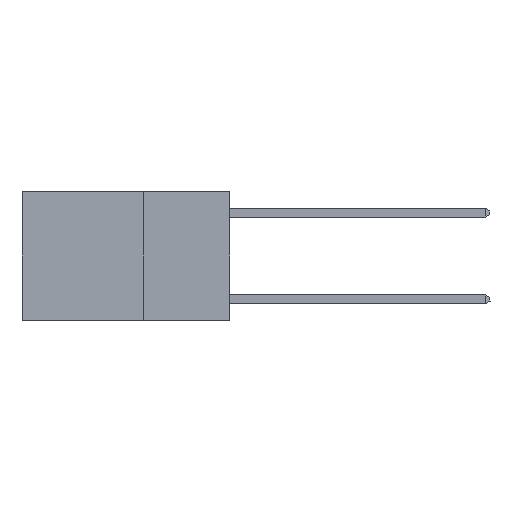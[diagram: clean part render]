
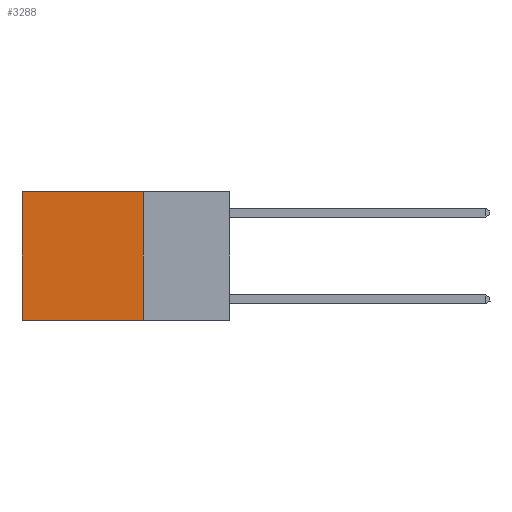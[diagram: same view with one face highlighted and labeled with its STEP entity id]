
A CAD part, left-side view. The second image highlights one B-rep face of the part: STEP entity #3288.
In plain terms, the highlighted planar face has unit normal (-1, 0, 0).
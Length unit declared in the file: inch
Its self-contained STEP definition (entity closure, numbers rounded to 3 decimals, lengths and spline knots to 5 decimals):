
#280 = CARTESIAN_POINT ( 'NONE',  ( 0.2625, 0.25, -0.37 ) ) ;
#695 = EDGE_LOOP ( 'NONE', ( #10145, #2868, #9260, #2559 ) ) ;
#1460 = LINE ( 'NONE', #3669, #13190 ) ;
#1894 = CARTESIAN_POINT ( 'NONE',  ( 0.2625, 0.6, -0.37 ) ) ;
#2559 = ORIENTED_EDGE ( 'NONE', *, *, #13387, .T. ) ;
#2843 = CARTESIAN_POINT ( 'NONE',  ( 0.2625, 0.6, 0. ) ) ;
#2868 = ORIENTED_EDGE ( 'NONE', *, *, #10816, .F. ) ;
#2948 = CARTESIAN_POINT ( 'NONE',  ( 0.2625, 0.25, -0.37 ) ) ;
#3288 = ADVANCED_FACE ( 'NONE', ( #13432 ), #14469, .F. ) ;
#3315 = CARTESIAN_POINT ( 'NONE',  ( 0.2625, 0.25, 0. ) ) ;
#3550 = VERTEX_POINT ( 'NONE', #12695 ) ;
#3669 = CARTESIAN_POINT ( 'NONE',  ( 0.2625, 0.25, 0. ) ) ;
#4218 = LINE ( 'NONE', #2843, #10522 ) ;
#4372 = VERTEX_POINT ( 'NONE', #10654 ) ;
#4763 = DIRECTION ( 'NONE',  ( 0., 1., 0. ) ) ;
#4798 = EDGE_CURVE ( 'NONE', #4372, #9120, #1460, .T. ) ;
#5135 = VECTOR ( 'NONE', #11990, 39.37008 ) ;
#5228 = LINE ( 'NONE', #13867, #12625 ) ;
#6815 = DIRECTION ( 'NONE',  ( 0., 0., -1. ) ) ;
#9120 = VERTEX_POINT ( 'NONE', #280 ) ;
#9260 = ORIENTED_EDGE ( 'NONE', *, *, #4798, .F. ) ;
#10145 = ORIENTED_EDGE ( 'NONE', *, *, #13495, .T. ) ;
#10522 = VECTOR ( 'NONE', #14108, 39.37008 ) ;
#10654 = CARTESIAN_POINT ( 'NONE',  ( 0.2625, 0.25, 0. ) ) ;
#10816 = EDGE_CURVE ( 'NONE', #9120, #11196, #13763, .T. ) ;
#11032 = DIRECTION ( 'NONE',  ( 1., 0., 0. ) ) ;
#11196 = VERTEX_POINT ( 'NONE', #1894 ) ;
#11704 = AXIS2_PLACEMENT_3D ( 'NONE', #3315, #11032, #12117 ) ;
#11990 = DIRECTION ( 'NONE',  ( 0., 1., 0. ) ) ;
#12117 = DIRECTION ( 'NONE',  ( 0., 0., -1. ) ) ;
#12625 = VECTOR ( 'NONE', #4763, 39.37008 ) ;
#12695 = CARTESIAN_POINT ( 'NONE',  ( 0.2625, 0.6, 0. ) ) ;
#13190 = VECTOR ( 'NONE', #6815, 39.37008 ) ;
#13387 = EDGE_CURVE ( 'NONE', #4372, #3550, #5228, .T. ) ;
#13432 = FACE_OUTER_BOUND ( 'NONE', #695, .T. ) ;
#13495 = EDGE_CURVE ( 'NONE', #3550, #11196, #4218, .T. ) ;
#13763 = LINE ( 'NONE', #2948, #5135 ) ;
#13867 = CARTESIAN_POINT ( 'NONE',  ( 0.2625, 0.25, 0. ) ) ;
#14108 = DIRECTION ( 'NONE',  ( 0., 0., -1. ) ) ;
#14469 = PLANE ( 'NONE',  #11704 ) ;
